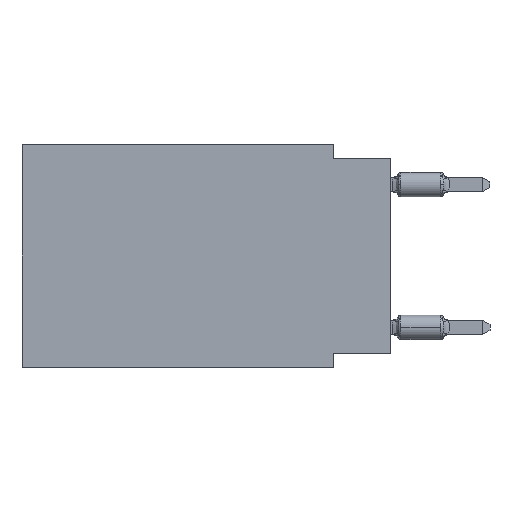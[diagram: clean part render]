
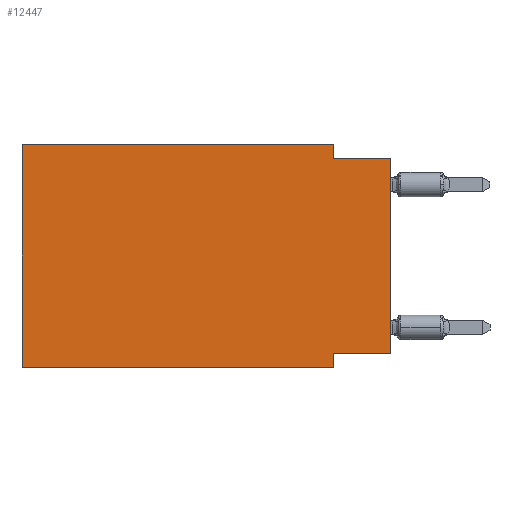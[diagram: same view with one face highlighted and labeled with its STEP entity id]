
A CAD part, left-side view. The second image highlights one B-rep face of the part: STEP entity #12447.
In plain terms, the highlighted planar face has unit normal (-1, 0, 0).
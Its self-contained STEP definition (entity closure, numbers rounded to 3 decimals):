
#29 = LINE ( 'NONE', #9786, #6807 ) ;
#197 = DIRECTION ( 'NONE',  ( 0., 0., 1. ) ) ;
#757 = VERTEX_POINT ( 'NONE', #8489 ) ;
#1228 = PLANE ( 'NONE',  #4084 ) ;
#1364 = VECTOR ( 'NONE', #8327, 1000. ) ;
#1614 = ORIENTED_EDGE ( 'NONE', *, *, #15410, .F. ) ;
#1968 = ORIENTED_EDGE ( 'NONE', *, *, #4383, .T. ) ;
#2135 = DIRECTION ( 'NONE',  ( 0., -1., 0. ) ) ;
#2216 = DIRECTION ( 'NONE',  ( 0., 0., -1. ) ) ;
#2249 = CARTESIAN_POINT ( 'NONE',  ( 0., 2.54, -0.635 ) ) ;
#3557 = CARTESIAN_POINT ( 'NONE',  ( 0., 16.383, -9.906 ) ) ;
#3656 = DIRECTION ( 'NONE',  ( 0., 0., -1. ) ) ;
#4084 = AXIS2_PLACEMENT_3D ( 'NONE', #13273, #12217, #2216 ) ;
#4328 = ORIENTED_EDGE ( 'NONE', *, *, #10678, .F. ) ;
#4383 = EDGE_CURVE ( 'NONE', #9142, #9548, #6343, .T. ) ;
#4794 = VERTEX_POINT ( 'NONE', #2249 ) ;
#5185 = EDGE_CURVE ( 'NONE', #4794, #9548, #14185, .T. ) ;
#5262 = DIRECTION ( 'NONE',  ( 0., 0., -1. ) ) ;
#5425 = LINE ( 'NONE', #15045, #13499 ) ;
#5877 = ORIENTED_EDGE ( 'NONE', *, *, #5908, .F. ) ;
#5908 = EDGE_CURVE ( 'NONE', #9142, #757, #8162, .T. ) ;
#6343 = LINE ( 'NONE', #11257, #15512 ) ;
#6556 = VECTOR ( 'NONE', #15422, 1000. ) ;
#6670 = VECTOR ( 'NONE', #2135, 1000. ) ;
#6807 = VECTOR ( 'NONE', #3656, 1000. ) ;
#6984 = CARTESIAN_POINT ( 'NONE',  ( 0., 16.383, 0. ) ) ;
#7043 = EDGE_CURVE ( 'NONE', #757, #12713, #29, .T. ) ;
#7135 = FACE_OUTER_BOUND ( 'NONE', #10402, .T. ) ;
#7201 = EDGE_CURVE ( 'NONE', #11296, #4794, #5425, .T. ) ;
#7438 = LINE ( 'NONE', #3557, #9744 ) ;
#7519 = LINE ( 'NONE', #6984, #6670 ) ;
#8056 = DIRECTION ( 'NONE',  ( 0., -1., 0. ) ) ;
#8101 = ORIENTED_EDGE ( 'NONE', *, *, #7201, .F. ) ;
#8162 = LINE ( 'NONE', #15503, #6556 ) ;
#8327 = DIRECTION ( 'NONE',  ( 0., 0., 1. ) ) ;
#8404 = CARTESIAN_POINT ( 'NONE',  ( 0., 16.383, 0. ) ) ;
#8482 = DIRECTION ( 'NONE',  ( 0., -1., 0. ) ) ;
#8489 = CARTESIAN_POINT ( 'NONE',  ( 0., 2.54, -9.271 ) ) ;
#9011 = CARTESIAN_POINT ( 'NONE',  ( 0., 0., -0.635 ) ) ;
#9092 = ORIENTED_EDGE ( 'NONE', *, *, #14158, .T. ) ;
#9142 = VERTEX_POINT ( 'NONE', #10759 ) ;
#9324 = VECTOR ( 'NONE', #8056, 1000. ) ;
#9548 = VERTEX_POINT ( 'NONE', #13396 ) ;
#9744 = VECTOR ( 'NONE', #8482, 1000. ) ;
#9786 = CARTESIAN_POINT ( 'NONE',  ( 0., 2.54, -9.906 ) ) ;
#10402 = EDGE_LOOP ( 'NONE', ( #1968, #10749, #8101, #1614, #4328, #9092, #14695, #5877 ) ) ;
#10678 = EDGE_CURVE ( 'NONE', #12901, #15674, #10897, .T. ) ;
#10749 = ORIENTED_EDGE ( 'NONE', *, *, #5185, .F. ) ;
#10759 = CARTESIAN_POINT ( 'NONE',  ( 0., 0., -9.271 ) ) ;
#10897 = LINE ( 'NONE', #8404, #1364 ) ;
#11030 = CARTESIAN_POINT ( 'NONE',  ( 0., 2.54, 0. ) ) ;
#11257 = CARTESIAN_POINT ( 'NONE',  ( 0., 0., 0. ) ) ;
#11296 = VERTEX_POINT ( 'NONE', #11030 ) ;
#12217 = DIRECTION ( 'NONE',  ( 1., 0., 0. ) ) ;
#12447 = ADVANCED_FACE ( 'NONE', ( #7135 ), #1228, .F. ) ;
#12713 = VERTEX_POINT ( 'NONE', #15518 ) ;
#12901 = VERTEX_POINT ( 'NONE', #13405 ) ;
#13273 = CARTESIAN_POINT ( 'NONE',  ( 0., 16.383, 0. ) ) ;
#13396 = CARTESIAN_POINT ( 'NONE',  ( 0., 0., -0.635 ) ) ;
#13405 = CARTESIAN_POINT ( 'NONE',  ( 0., 16.383, -9.906 ) ) ;
#13499 = VECTOR ( 'NONE', #5262, 1000. ) ;
#14158 = EDGE_CURVE ( 'NONE', #12901, #12713, #7438, .T. ) ;
#14185 = LINE ( 'NONE', #9011, #9324 ) ;
#14695 = ORIENTED_EDGE ( 'NONE', *, *, #7043, .F. ) ;
#15045 = CARTESIAN_POINT ( 'NONE',  ( 0., 2.54, 0. ) ) ;
#15410 = EDGE_CURVE ( 'NONE', #15674, #11296, #7519, .T. ) ;
#15422 = DIRECTION ( 'NONE',  ( 0., 1., 0. ) ) ;
#15503 = CARTESIAN_POINT ( 'NONE',  ( 0., 0., -9.271 ) ) ;
#15512 = VECTOR ( 'NONE', #197, 1000. ) ;
#15518 = CARTESIAN_POINT ( 'NONE',  ( 0., 2.54, -9.906 ) ) ;
#15674 = VERTEX_POINT ( 'NONE', #15884 ) ;
#15884 = CARTESIAN_POINT ( 'NONE',  ( 0., 16.383, 0. ) ) ;
